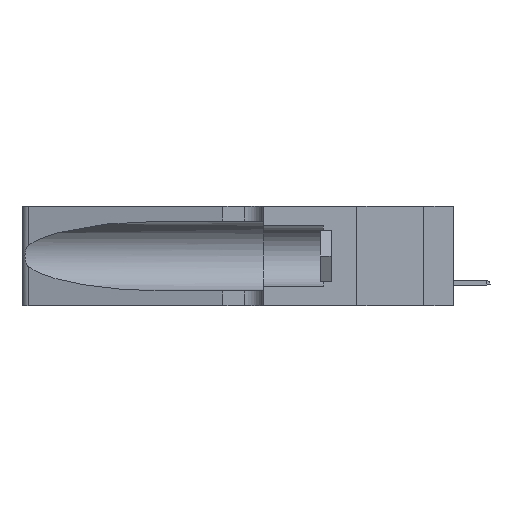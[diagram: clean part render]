
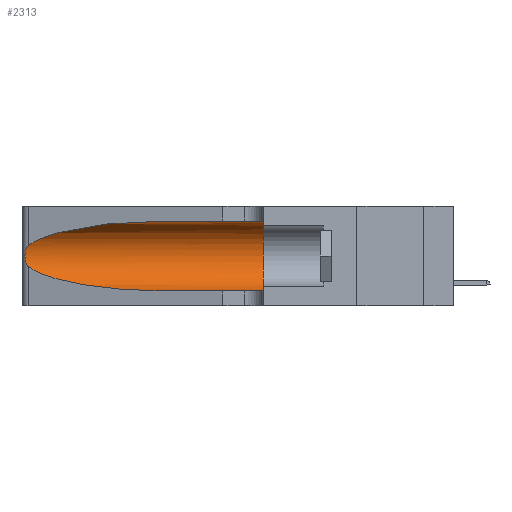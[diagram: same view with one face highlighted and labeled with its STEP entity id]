
A CAD part, left-side view. The second image highlights one B-rep face of the part: STEP entity #2313.
In plain terms, the highlighted cylindrical face has radius 3.308 mm (diameter 6.617 mm), a partial arc.
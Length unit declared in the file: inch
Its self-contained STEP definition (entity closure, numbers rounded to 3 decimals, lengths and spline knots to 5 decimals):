
#205 = CARTESIAN_POINT ( 'NONE',  ( 0.2373, 1.15595, 0.28018 ) ) ;
#826 = CARTESIAN_POINT ( 'NONE',  ( 0.1305, 0.35, 0.31525 ) ) ;
#1528 = DIRECTION ( 'NONE',  ( 0., -1., 0. ) ) ;
#1742 = CARTESIAN_POINT ( 'NONE',  ( 0.25487, 1.22718, 0.14631 ) ) ;
#1888 = CARTESIAN_POINT ( 'NONE',  ( 0.2373, 1.15595, 0.08982 ) ) ;
#2195 = AXIS2_PLACEMENT_3D ( 'NONE', #5653, #13089, #7476 ) ;
#2271 = CARTESIAN_POINT ( 'NONE',  ( 0.18966, 0.96281, 0.31525 ) ) ;
#2313 = ADVANCED_FACE ( 'NONE', ( #15701 ), #8244, .F. ) ;
#2598 = EDGE_CURVE ( 'NONE', #11196, #11149, #13491, .T. ) ;
#2678 = ORIENTED_EDGE ( 'NONE', *, *, #23562, .T. ) ;
#3235 = CARTESIAN_POINT ( 'NONE',  ( 0.26075, 1.23896, 0.19203 ) ) ;
#3835 = CARTESIAN_POINT ( 'NONE',  ( 0.18966, 0.96281, 0.05475 ) ) ;
#4589 = CARTESIAN_POINT ( 'NONE',  ( 0.1305, 1.61858, 0.185 ) ) ;
#4695 = CARTESIAN_POINT ( 'NONE',  ( 0.25639, 1.23184, 0.21858 ) ) ;
#5653 = CARTESIAN_POINT ( 'NONE',  ( 0.1305, 0.35, 0.185 ) ) ;
#5702 = VERTEX_POINT ( 'NONE', #21444 ) ;
#6295 = CARTESIAN_POINT ( 'NONE',  ( 0.1305, 1.61858, 0.31525 ) ) ;
#6676 = VERTEX_POINT ( 'NONE', #8535 ) ;
#6715 = EDGE_LOOP ( 'NONE', ( #13867, #7169, #18657, #2678, #21145, #16282 ) ) ;
#7169 = ORIENTED_EDGE ( 'NONE', *, *, #20913, .T. ) ;
#7211 = CIRCLE ( 'NONE', #2195, 0.13025 ) ;
#7420 = VERTEX_POINT ( 'NONE', #826 ) ;
#7476 = DIRECTION ( 'NONE',  ( 0., 0., 1. ) ) ;
#7987 = CARTESIAN_POINT ( 'NONE',  ( 0.25487, 1.22718, 0.22369 ) ) ;
#8244 = CYLINDRICAL_SURFACE ( 'NONE', #19105, 0.13025 ) ;
#8535 = CARTESIAN_POINT ( 'NONE',  ( 0.25487, 1.22718, 0.22369 ) ) ;
#8694 = CARTESIAN_POINT ( 'NONE',  ( 0.25789, 1.23486, 0.15765 ) ) ;
#10522 = CARTESIAN_POINT ( 'NONE',  ( 0.25487, 1.22718, 0.22369 ) ) ;
#10531 = LINE ( 'NONE', #23956, #12830 ) ;
#10620 = EDGE_CURVE ( 'NONE', #5702, #7420, #13605, .T. ) ;
#10760 = CARTESIAN_POINT ( 'NONE',  ( 0.25555, 1.22993, 0.14849 ) ) ;
#11149 = VERTEX_POINT ( 'NONE', #15768 ) ;
#11196 = VERTEX_POINT ( 'NONE', #1742 ) ;
#11906 = DIRECTION ( 'NONE',  ( 0., -1., 0. ) ) ;
#12307 = VERTEX_POINT ( 'NONE', #20660 ) ;
#12830 = VECTOR ( 'NONE', #1528, 39.37008 ) ;
#13089 = DIRECTION ( 'NONE',  ( 0., 1., 0. ) ) ;
#13491 =( BOUNDED_CURVE ( )  B_SPLINE_CURVE ( 3, ( #20801, #1888, #3835, #18723 ),
 .UNSPECIFIED., .F., .F. ) 
 B_SPLINE_CURVE_WITH_KNOTS ( ( 4, 4 ),
 ( 3.44316, 4.71239 ),
 .UNSPECIFIED. ) 
 CURVE ( )  GEOMETRIC_REPRESENTATION_ITEM ( )  RATIONAL_B_SPLINE_CURVE ( ( 1., 0.87, 0.87, 1. ) ) 
 REPRESENTATION_ITEM ( '' )  );
#13494 = CARTESIAN_POINT ( 'NONE',  ( 0.1305, 0.72297, 0.31525 ) ) ;
#13605 = LINE ( 'NONE', #6295, #18281 ) ;
#13867 = ORIENTED_EDGE ( 'NONE', *, *, #15224, .T. ) ;
#14198 = CARTESIAN_POINT ( 'NONE',  ( 0.25856, 1.23593, 0.16098 ) ) ;
#14431 = CARTESIAN_POINT ( 'NONE',  ( 0.25787, 1.23484, 0.2124 ) ) ;
#15224 = EDGE_CURVE ( 'NONE', #5702, #6676, #20335, .T. ) ;
#15701 = FACE_OUTER_BOUND ( 'NONE', #6715, .T. ) ;
#15768 = CARTESIAN_POINT ( 'NONE',  ( 0.1305, 0.72297, 0.05475 ) ) ;
#16031 = CARTESIAN_POINT ( 'NONE',  ( 0.26017, 1.23833, 0.17102 ) ) ;
#16282 = ORIENTED_EDGE ( 'NONE', *, *, #10620, .F. ) ;
#17975 = CARTESIAN_POINT ( 'NONE',  ( 0.25854, 1.2359, 0.20912 ) ) ;
#18092 = CARTESIAN_POINT ( 'NONE',  ( 0.26075, 1.23896, 0.178 ) ) ;
#18211 = B_SPLINE_CURVE_WITH_KNOTS ( 'NONE', 3,
 ( #10522, #21753, #4695, #14431, #17975, #23706, #3235, #18092, #16031, #14198, #8694, #19806, #10760, #21880 ),
 .UNSPECIFIED., .F., .F.,
 ( 4, 2, 2, 2, 2, 2, 4 ),
 ( 0., 0.00027, 0.00053, 0.00107, 0.0016, 0.00187, 0.00214 ),
 .UNSPECIFIED. ) ;
#18281 = VECTOR ( 'NONE', #11906, 39.37008 ) ;
#18657 = ORIENTED_EDGE ( 'NONE', *, *, #2598, .T. ) ;
#18723 = CARTESIAN_POINT ( 'NONE',  ( 0.1305, 0.72297, 0.05475 ) ) ;
#19105 = AXIS2_PLACEMENT_3D ( 'NONE', #4589, #19118, #22895 ) ;
#19118 = DIRECTION ( 'NONE',  ( 0., -1., 0. ) ) ;
#19806 = CARTESIAN_POINT ( 'NONE',  ( 0.25639, 1.23186, 0.15144 ) ) ;
#19824 = EDGE_CURVE ( 'NONE', #7420, #12307, #7211, .T. ) ;
#20335 =( BOUNDED_CURVE ( )  B_SPLINE_CURVE ( 3, ( #13494, #2271, #205, #7987 ),
 .UNSPECIFIED., .F., .T. ) 
 B_SPLINE_CURVE_WITH_KNOTS ( ( 4, 4 ),
 ( 1.5708, 2.84003 ),
 .UNSPECIFIED. ) 
 CURVE ( )  GEOMETRIC_REPRESENTATION_ITEM ( )  RATIONAL_B_SPLINE_CURVE ( ( 1., 0.87, 0.87, 1. ) ) 
 REPRESENTATION_ITEM ( '' )  );
#20660 = CARTESIAN_POINT ( 'NONE',  ( 0.1305, 0.35, 0.05475 ) ) ;
#20801 = CARTESIAN_POINT ( 'NONE',  ( 0.25487, 1.22718, 0.14631 ) ) ;
#20913 = EDGE_CURVE ( 'NONE', #6676, #11196, #18211, .T. ) ;
#21145 = ORIENTED_EDGE ( 'NONE', *, *, #19824, .F. ) ;
#21444 = CARTESIAN_POINT ( 'NONE',  ( 0.1305, 0.72297, 0.31525 ) ) ;
#21753 = CARTESIAN_POINT ( 'NONE',  ( 0.25555, 1.22994, 0.2215 ) ) ;
#21880 = CARTESIAN_POINT ( 'NONE',  ( 0.25487, 1.22718, 0.14631 ) ) ;
#22895 = DIRECTION ( 'NONE',  ( 0., 0., -1. ) ) ;
#23562 = EDGE_CURVE ( 'NONE', #11149, #12307, #10531, .T. ) ;
#23706 = CARTESIAN_POINT ( 'NONE',  ( 0.26018, 1.23835, 0.19895 ) ) ;
#23956 = CARTESIAN_POINT ( 'NONE',  ( 0.1305, 1.61858, 0.05475 ) ) ;
